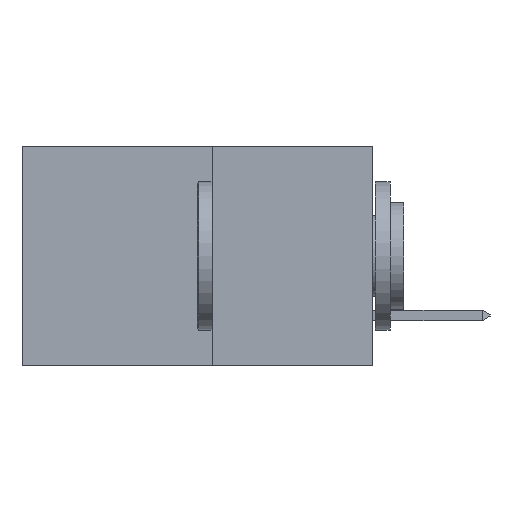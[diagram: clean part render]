
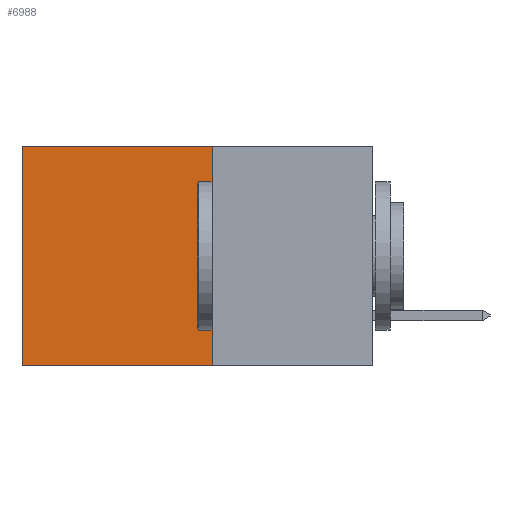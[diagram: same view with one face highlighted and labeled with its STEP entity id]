
A CAD part, left-side view. The second image highlights one B-rep face of the part: STEP entity #6988.
In plain terms, the highlighted planar face has unit normal (-1, 0, 0).
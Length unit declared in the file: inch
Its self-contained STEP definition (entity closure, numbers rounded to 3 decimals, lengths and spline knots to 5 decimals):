
#394 = EDGE_CURVE ( 'NONE', #12358, #21828, #5566, .T. ) ;
#1142 = CARTESIAN_POINT ( 'NONE',  ( 0.277, 0.27, 0. ) ) ;
#1351 = EDGE_CURVE ( 'NONE', #23502, #12358, #7731, .T. ) ;
#3964 = DIRECTION ( 'NONE',  ( 0., 0., -1. ) ) ;
#4222 = VECTOR ( 'NONE', #9851, 39.37008 ) ;
#5504 = LINE ( 'NONE', #8590, #6138 ) ;
#5566 = LINE ( 'NONE', #15339, #16268 ) ;
#5587 = VERTEX_POINT ( 'NONE', #9436 ) ;
#6138 = VECTOR ( 'NONE', #22764, 39.37008 ) ;
#6988 = ADVANCED_FACE ( 'NONE', ( #9739 ), #7154, .F. ) ;
#7154 = PLANE ( 'NONE',  #22883 ) ;
#7155 = LINE ( 'NONE', #23093, #22649 ) ;
#7731 = LINE ( 'NONE', #1142, #4222 ) ;
#8590 = CARTESIAN_POINT ( 'NONE',  ( 0.277, 0.27, -0.37 ) ) ;
#9436 = CARTESIAN_POINT ( 'NONE',  ( 0.277, 0.27, -0.37 ) ) ;
#9739 = FACE_OUTER_BOUND ( 'NONE', #22026, .T. ) ;
#9851 = DIRECTION ( 'NONE',  ( 0., 1., 0. ) ) ;
#10927 = DIRECTION ( 'NONE',  ( 0., 0., -1. ) ) ;
#11182 = DIRECTION ( 'NONE',  ( 1., 0., 0. ) ) ;
#12358 = VERTEX_POINT ( 'NONE', #21490 ) ;
#15339 = CARTESIAN_POINT ( 'NONE',  ( 0.277, 0.59, -0.37 ) ) ;
#16268 = VECTOR ( 'NONE', #3964, 39.37008 ) ;
#18150 = ORIENTED_EDGE ( 'NONE', *, *, #1351, .T. ) ;
#18315 = EDGE_CURVE ( 'NONE', #23502, #5587, #7155, .T. ) ;
#19257 = CARTESIAN_POINT ( 'NONE',  ( 0.277, 0.59, -0.37 ) ) ;
#19458 = EDGE_CURVE ( 'NONE', #5587, #21828, #5504, .T. ) ;
#20936 = CARTESIAN_POINT ( 'NONE',  ( 0.277, 0.27, 0. ) ) ;
#21030 = ORIENTED_EDGE ( 'NONE', *, *, #19458, .F. ) ;
#21490 = CARTESIAN_POINT ( 'NONE',  ( 0.277, 0.59, 0. ) ) ;
#21828 = VERTEX_POINT ( 'NONE', #19257 ) ;
#22026 = EDGE_LOOP ( 'NONE', ( #25781, #21030, #22940, #18150 ) ) ;
#22649 = VECTOR ( 'NONE', #10927, 39.37008 ) ;
#22764 = DIRECTION ( 'NONE',  ( 0., 1., 0. ) ) ;
#22883 = AXIS2_PLACEMENT_3D ( 'NONE', #23341, #11182, #25367 ) ;
#22940 = ORIENTED_EDGE ( 'NONE', *, *, #18315, .F. ) ;
#23093 = CARTESIAN_POINT ( 'NONE',  ( 0.277, 0.27, -0.37 ) ) ;
#23341 = CARTESIAN_POINT ( 'NONE',  ( 0.277, 0.27, -0.37 ) ) ;
#23502 = VERTEX_POINT ( 'NONE', #20936 ) ;
#25367 = DIRECTION ( 'NONE',  ( 0., 0., -1. ) ) ;
#25781 = ORIENTED_EDGE ( 'NONE', *, *, #394, .T. ) ;
